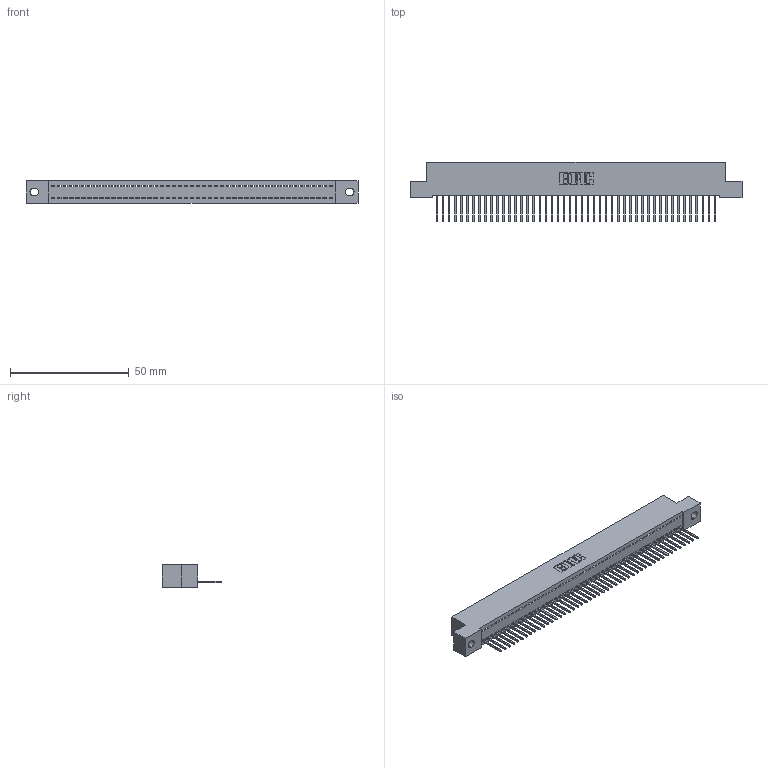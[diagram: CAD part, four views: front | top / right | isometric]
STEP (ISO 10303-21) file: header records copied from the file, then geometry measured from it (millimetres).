
FILE_DESCRIPTION (( 'STEP AP203' ), '1' );
FILE_NAME ('342-047-523-102.STEP', '2018-08-12T16:58:34', ( '' ), ( '' ), 'SwSTEP 2.0', 'SolidWorks 2016', '' );
FILE_SCHEMA (( 'CONFIG_CONTROL_DESIGN' ));
Length unit declared in the file: inch
Products named in the file (3): 342 Part_.128 Slot; 345-292-001_345-293-123; 342-047-523-102
Assembly tree (48 placements, depth 2):
  342-047-523-102
    342 Part_.128 Slot
    345-292-001_345-293-123  x47
Bounding box: 139.7 x 25.15 x 9.4 mm (x, y, z)
Volume: 12197 mm3; surface area: 17808.5 mm2
Topology: 48 solids, 48 shells, 2840 faces, 8583 edges, 5658 vertices
Faces by surface type: plane 2044, cylinder 796
Entity records: 28107 total; most frequent: CARTESIAN_POINT 4855, ORIENTED_EDGE 4838, DIRECTION 4085, EDGE_CURVE 2419, VECTOR 2291, LINE 2291, VERTEX_POINT 1610, AXIS2_PLACEMENT_3D 897
